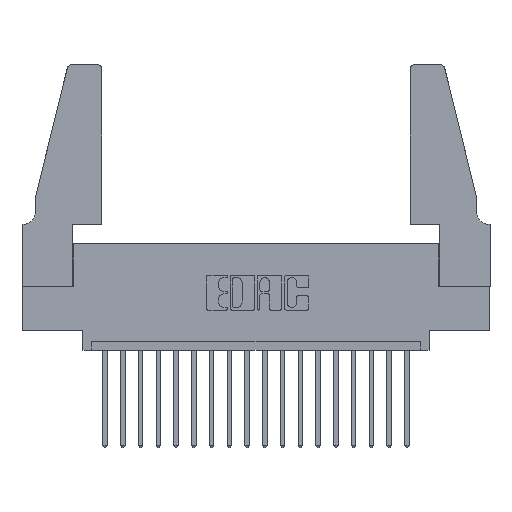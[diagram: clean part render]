
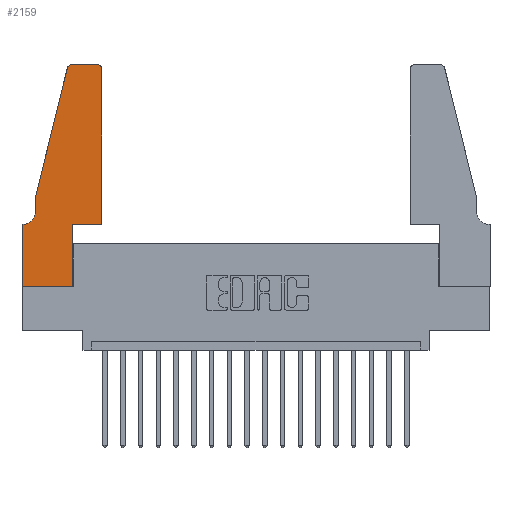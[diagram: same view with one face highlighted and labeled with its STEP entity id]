
A CAD part, top view. The second image highlights one B-rep face of the part: STEP entity #2159.
In plain terms, the highlighted planar face has unit normal (0, 0, 1).
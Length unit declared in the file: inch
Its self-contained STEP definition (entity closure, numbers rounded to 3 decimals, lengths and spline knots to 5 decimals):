
#50 = EDGE_CURVE ( 'NONE', #7414, #1392, #14167, .T. ) ;
#93 = CARTESIAN_POINT ( 'NONE',  ( 0.4505, 1.22, 0.37 ) ) ;
#357 = CARTESIAN_POINT ( 'NONE',  ( 0., 0.35, 0.37 ) ) ;
#1392 = VERTEX_POINT ( 'NONE', #5906 ) ;
#1429 = ORIENTED_EDGE ( 'NONE', *, *, #1892, .T. ) ;
#1536 = ORIENTED_EDGE ( 'NONE', *, *, #8888, .T. ) ;
#1847 = DIRECTION ( 'NONE',  ( 0., 0., 1. ) ) ;
#1892 = EDGE_CURVE ( 'NONE', #13985, #8387, #3992, .T. ) ;
#2138 = EDGE_LOOP ( 'NONE', ( #1536, #18479, #2447, #1429, #16472, #18286, #4681, #10938, #2300, #10248, #3269, #15539 ) ) ;
#2159 = ADVANCED_FACE ( 'NONE', ( #17555 ), #10906, .T. ) ;
#2201 = LINE ( 'NONE', #18037, #5151 ) ;
#2248 = DIRECTION ( 'NONE',  ( -0.239, -0.971, 0. ) ) ;
#2300 = ORIENTED_EDGE ( 'NONE', *, *, #7724, .T. ) ;
#2447 = ORIENTED_EDGE ( 'NONE', *, *, #15952, .T. ) ;
#2777 = EDGE_CURVE ( 'NONE', #7924, #16723, #18450, .T. ) ;
#2911 = VECTOR ( 'NONE', #6584, 39.37008 ) ;
#3134 = DIRECTION ( 'NONE',  ( 1., 0., 0. ) ) ;
#3269 = ORIENTED_EDGE ( 'NONE', *, *, #10919, .T. ) ;
#3992 = LINE ( 'NONE', #13433, #7902 ) ;
#4231 = CARTESIAN_POINT ( 'NONE',  ( 0.0755, 0.42, 0.37 ) ) ;
#4316 = LINE ( 'NONE', #7562, #13954 ) ;
#4349 = DIRECTION ( 'NONE',  ( -1., 0., 0. ) ) ;
#4444 = DIRECTION ( 'NONE',  ( 1., 0., 0. ) ) ;
#4528 = EDGE_CURVE ( 'NONE', #8387, #16240, #4786, .T. ) ;
#4643 = DIRECTION ( 'NONE',  ( 0., -1., 0. ) ) ;
#4681 = ORIENTED_EDGE ( 'NONE', *, *, #14166, .T. ) ;
#4786 = CIRCLE ( 'NONE', #4863, 0.07 ) ;
#4797 = DIRECTION ( 'NONE',  ( 0., 1., 0. ) ) ;
#4863 = AXIS2_PLACEMENT_3D ( 'NONE', #13810, #16558, #7708 ) ;
#5091 = CARTESIAN_POINT ( 'NONE',  ( 0.4505, 0.35, 0.37 ) ) ;
#5109 = LINE ( 'NONE', #15950, #16357 ) ;
#5138 = VERTEX_POINT ( 'NONE', #8803 ) ;
#5151 = VECTOR ( 'NONE', #10599, 39.37008 ) ;
#5906 = CARTESIAN_POINT ( 'NONE',  ( 0.2865, 0., 0.37 ) ) ;
#6278 = AXIS2_PLACEMENT_3D ( 'NONE', #12558, #15681, #18397 ) ;
#6310 = CARTESIAN_POINT ( 'NONE',  ( 0.4205, 1.25, 0.37 ) ) ;
#6317 = VERTEX_POINT ( 'NONE', #357 ) ;
#6477 = CARTESIAN_POINT ( 'NONE',  ( 0.0755, 0.5, 0.37 ) ) ;
#6584 = DIRECTION ( 'NONE',  ( 1., 0., 0. ) ) ;
#6865 = EDGE_CURVE ( 'NONE', #16240, #6317, #10801, .T. ) ;
#7193 = EDGE_CURVE ( 'NONE', #14379, #7246, #14654, .T. ) ;
#7246 = VERTEX_POINT ( 'NONE', #18930 ) ;
#7366 = LINE ( 'NONE', #18158, #18633 ) ;
#7414 = VERTEX_POINT ( 'NONE', #17145 ) ;
#7562 = CARTESIAN_POINT ( 'NONE',  ( 0.2865, 0.35, 0.37 ) ) ;
#7572 = CARTESIAN_POINT ( 'NONE',  ( 0.4205, 1.22, 0.37 ) ) ;
#7708 = DIRECTION ( 'NONE',  ( -1., 0., 0. ) ) ;
#7724 = EDGE_CURVE ( 'NONE', #1392, #14379, #4316, .T. ) ;
#7902 = VECTOR ( 'NONE', #4643, 39.37008 ) ;
#7924 = VERTEX_POINT ( 'NONE', #93 ) ;
#7967 = LINE ( 'NONE', #14550, #14621 ) ;
#8263 = CARTESIAN_POINT ( 'NONE',  ( 0.2865, 0.35, 0.37 ) ) ;
#8387 = VERTEX_POINT ( 'NONE', #4231 ) ;
#8803 = CARTESIAN_POINT ( 'NONE',  ( 0.284, 1.25, 0.37 ) ) ;
#8888 = EDGE_CURVE ( 'NONE', #16723, #5138, #7967, .T. ) ;
#8935 = DIRECTION ( 'NONE',  ( 1., 0., 0. ) ) ;
#9361 = DIRECTION ( 'NONE',  ( 0., 1., 0. ) ) ;
#10248 = ORIENTED_EDGE ( 'NONE', *, *, #7193, .T. ) ;
#10373 = VERTEX_POINT ( 'NONE', #19110 ) ;
#10599 = DIRECTION ( 'NONE',  ( 0., -1., 0. ) ) ;
#10624 = CARTESIAN_POINT ( 'NONE',  ( 0.0055, 0.35, 0.37 ) ) ;
#10801 = LINE ( 'NONE', #13348, #13279 ) ;
#10906 = PLANE ( 'NONE',  #6278 ) ;
#10919 = EDGE_CURVE ( 'NONE', #7246, #7924, #5109, .T. ) ;
#10938 = ORIENTED_EDGE ( 'NONE', *, *, #50, .T. ) ;
#12558 = CARTESIAN_POINT ( 'NONE',  ( 0., 0.35, 0.37 ) ) ;
#13279 = VECTOR ( 'NONE', #14842, 39.37008 ) ;
#13348 = CARTESIAN_POINT ( 'NONE',  ( 0.0755, 0.35, 0.37 ) ) ;
#13413 = DIRECTION ( 'NONE',  ( 0., 0., 1. ) ) ;
#13433 = CARTESIAN_POINT ( 'NONE',  ( 0.0755, 0.5, 0.37 ) ) ;
#13740 = VECTOR ( 'NONE', #8935, 39.37008 ) ;
#13810 = CARTESIAN_POINT ( 'NONE',  ( 0.0055, 0.42, 0.37 ) ) ;
#13954 = VECTOR ( 'NONE', #4797, 39.37008 ) ;
#13985 = VERTEX_POINT ( 'NONE', #6477 ) ;
#14166 = EDGE_CURVE ( 'NONE', #6317, #7414, #2201, .T. ) ;
#14167 = LINE ( 'NONE', #15344, #2911 ) ;
#14379 = VERTEX_POINT ( 'NONE', #8263 ) ;
#14550 = CARTESIAN_POINT ( 'NONE',  ( 0.2605, 1.25, 0.37 ) ) ;
#14621 = VECTOR ( 'NONE', #4349, 39.37008 ) ;
#14654 = LINE ( 'NONE', #5091, #13740 ) ;
#14679 = AXIS2_PLACEMENT_3D ( 'NONE', #7572, #13413, #4444 ) ;
#14842 = DIRECTION ( 'NONE',  ( -1., 0., 0. ) ) ;
#14942 = AXIS2_PLACEMENT_3D ( 'NONE', #16462, #1847, #3134 ) ;
#15344 = CARTESIAN_POINT ( 'NONE',  ( 0., 0., 0.37 ) ) ;
#15539 = ORIENTED_EDGE ( 'NONE', *, *, #2777, .T. ) ;
#15681 = DIRECTION ( 'NONE',  ( 0., 0., 1. ) ) ;
#15702 = EDGE_CURVE ( 'NONE', #5138, #10373, #16560, .T. ) ;
#15950 = CARTESIAN_POINT ( 'NONE',  ( 0.4505, 0.35, 0.37 ) ) ;
#15952 = EDGE_CURVE ( 'NONE', #10373, #13985, #7366, .T. ) ;
#16240 = VERTEX_POINT ( 'NONE', #10624 ) ;
#16357 = VECTOR ( 'NONE', #9361, 39.37008 ) ;
#16462 = CARTESIAN_POINT ( 'NONE',  ( 0.284, 1.22, 0.37 ) ) ;
#16472 = ORIENTED_EDGE ( 'NONE', *, *, #4528, .T. ) ;
#16558 = DIRECTION ( 'NONE',  ( 0., 0., -1. ) ) ;
#16560 = CIRCLE ( 'NONE', #14942, 0.03 ) ;
#16723 = VERTEX_POINT ( 'NONE', #6310 ) ;
#17145 = CARTESIAN_POINT ( 'NONE',  ( 0., 0., 0.37 ) ) ;
#17555 = FACE_OUTER_BOUND ( 'NONE', #2138, .T. ) ;
#18037 = CARTESIAN_POINT ( 'NONE',  ( 0., 0., 0.37 ) ) ;
#18158 = CARTESIAN_POINT ( 'NONE',  ( 0.0755, 0.5, 0.37 ) ) ;
#18286 = ORIENTED_EDGE ( 'NONE', *, *, #6865, .T. ) ;
#18397 = DIRECTION ( 'NONE',  ( 1., 0., 0. ) ) ;
#18450 = CIRCLE ( 'NONE', #14679, 0.03 ) ;
#18479 = ORIENTED_EDGE ( 'NONE', *, *, #15702, .T. ) ;
#18633 = VECTOR ( 'NONE', #2248, 39.37008 ) ;
#18930 = CARTESIAN_POINT ( 'NONE',  ( 0.4505, 0.35, 0.37 ) ) ;
#19110 = CARTESIAN_POINT ( 'NONE',  ( 0.25487, 1.22718, 0.37 ) ) ;
